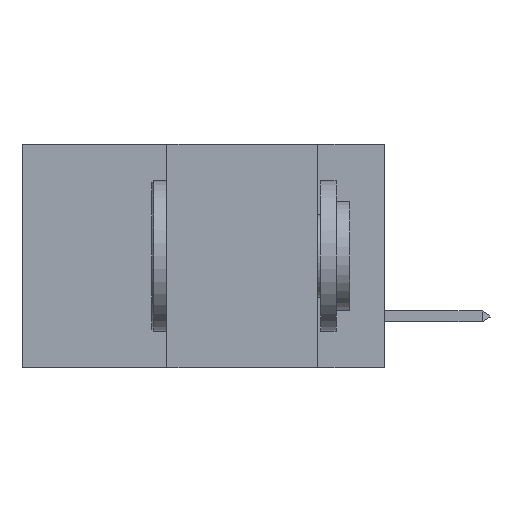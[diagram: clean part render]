
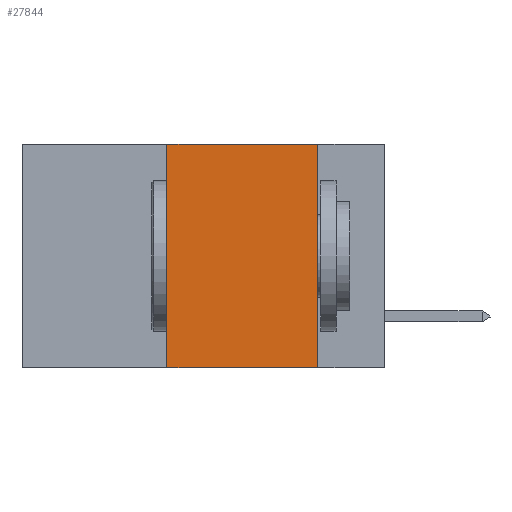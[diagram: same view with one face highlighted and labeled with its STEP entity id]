
A CAD part, left-side view. The second image highlights one B-rep face of the part: STEP entity #27844.
In plain terms, the highlighted planar face has unit normal (-1, 0, 0).
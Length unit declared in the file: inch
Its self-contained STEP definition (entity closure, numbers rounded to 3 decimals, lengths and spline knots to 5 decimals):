
#1611 = CARTESIAN_POINT ( 'NONE',  ( 0., 0.6, 0. ) ) ;
#1740 = VERTEX_POINT ( 'NONE', #43828 ) ;
#4299 = EDGE_CURVE ( 'NONE', #6921, #1740, #45383, .T. ) ;
#5598 = EDGE_LOOP ( 'NONE', ( #28529, #8126, #22020, #29932 ) ) ;
#6921 = VERTEX_POINT ( 'NONE', #40441 ) ;
#8126 = ORIENTED_EDGE ( 'NONE', *, *, #21899, .F. ) ;
#9490 = CARTESIAN_POINT ( 'NONE',  ( 0., 0.36, -0.37 ) ) ;
#11459 = VECTOR ( 'NONE', #39768, 39.37008 ) ;
#13411 = FACE_OUTER_BOUND ( 'NONE', #5598, .T. ) ;
#13541 = AXIS2_PLACEMENT_3D ( 'NONE', #1611, #19971, #27506 ) ;
#14997 = LINE ( 'NONE', #19065, #20917 ) ;
#16465 = EDGE_CURVE ( 'NONE', #39347, #35953, #34341, .T. ) ;
#17391 = CARTESIAN_POINT ( 'NONE',  ( 0., 0.36, 0. ) ) ;
#19065 = CARTESIAN_POINT ( 'NONE',  ( 0., 0.6, 0. ) ) ;
#19971 = DIRECTION ( 'NONE',  ( 1., 0., 0. ) ) ;
#20917 = VECTOR ( 'NONE', #38407, 39.37008 ) ;
#21899 = EDGE_CURVE ( 'NONE', #35953, #6921, #14997, .T. ) ;
#22020 = ORIENTED_EDGE ( 'NONE', *, *, #16465, .F. ) ;
#23749 = VECTOR ( 'NONE', #24060, 39.37008 ) ;
#24060 = DIRECTION ( 'NONE',  ( 0., -1., 0. ) ) ;
#27506 = DIRECTION ( 'NONE',  ( 0., 0., -1. ) ) ;
#27844 = ADVANCED_FACE ( 'NONE', ( #13411 ), #46883, .F. ) ;
#28529 = ORIENTED_EDGE ( 'NONE', *, *, #4299, .F. ) ;
#29932 = ORIENTED_EDGE ( 'NONE', *, *, #45631, .T. ) ;
#31578 = CARTESIAN_POINT ( 'NONE',  ( 0., 0.36, 0. ) ) ;
#32491 = VECTOR ( 'NONE', #44916, 39.37008 ) ;
#34341 = LINE ( 'NONE', #17391, #11459 ) ;
#35425 = CARTESIAN_POINT ( 'NONE',  ( 0., 0.6, -0.37 ) ) ;
#35953 = VERTEX_POINT ( 'NONE', #31578 ) ;
#36745 = LINE ( 'NONE', #35425, #23749 ) ;
#38407 = DIRECTION ( 'NONE',  ( 0., -1., 0. ) ) ;
#39347 = VERTEX_POINT ( 'NONE', #9490 ) ;
#39768 = DIRECTION ( 'NONE',  ( 0., 0., 1. ) ) ;
#40441 = CARTESIAN_POINT ( 'NONE',  ( 0., 0.11, 0. ) ) ;
#43828 = CARTESIAN_POINT ( 'NONE',  ( 0., 0.11, -0.37 ) ) ;
#44916 = DIRECTION ( 'NONE',  ( 0., 0., -1. ) ) ;
#45383 = LINE ( 'NONE', #48400, #32491 ) ;
#45631 = EDGE_CURVE ( 'NONE', #39347, #1740, #36745, .T. ) ;
#46883 = PLANE ( 'NONE',  #13541 ) ;
#48400 = CARTESIAN_POINT ( 'NONE',  ( 0., 0.11, 0. ) ) ;
